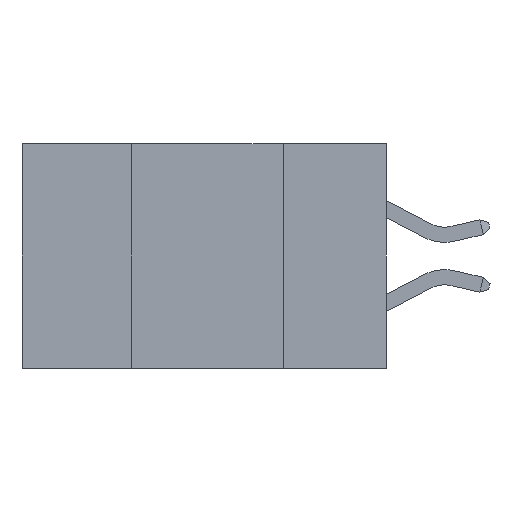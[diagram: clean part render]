
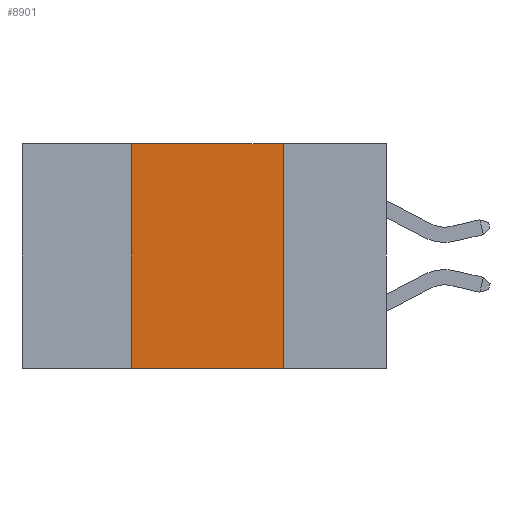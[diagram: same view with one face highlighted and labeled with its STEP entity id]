
A CAD part, left-side view. The second image highlights one B-rep face of the part: STEP entity #8901.
In plain terms, the highlighted planar face has unit normal (-1, 0, 0).
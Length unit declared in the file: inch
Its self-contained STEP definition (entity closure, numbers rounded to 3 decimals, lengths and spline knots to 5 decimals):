
#100 = DIRECTION ( 'NONE',  ( 0., -1., 0. ) ) ;
#317 = EDGE_LOOP ( 'NONE', ( #9134, #7067, #1886, #10419 ) ) ;
#601 = VERTEX_POINT ( 'NONE', #1994 ) ;
#633 = DIRECTION ( 'NONE',  ( 1., 0., 0. ) ) ;
#778 = VERTEX_POINT ( 'NONE', #4035 ) ;
#921 = VERTEX_POINT ( 'NONE', #9400 ) ;
#1886 = ORIENTED_EDGE ( 'NONE', *, *, #10093, .F. ) ;
#1994 = CARTESIAN_POINT ( 'NONE',  ( 0., 0.17, 0. ) ) ;
#2446 = CARTESIAN_POINT ( 'NONE',  ( 0., 0.42, -0.37 ) ) ;
#3532 = LINE ( 'NONE', #3844, #10837 ) ;
#3844 = CARTESIAN_POINT ( 'NONE',  ( 0., 0.6, -0.37 ) ) ;
#4035 = CARTESIAN_POINT ( 'NONE',  ( 0., 0.42, 0. ) ) ;
#5699 = CARTESIAN_POINT ( 'NONE',  ( 0., 0.6, 0. ) ) ;
#5722 = FACE_OUTER_BOUND ( 'NONE', #317, .T. ) ;
#5918 = EDGE_CURVE ( 'NONE', #6959, #921, #3532, .T. ) ;
#6034 = EDGE_CURVE ( 'NONE', #601, #921, #12149, .T. ) ;
#6339 = CARTESIAN_POINT ( 'NONE',  ( 0., 0.6, 0. ) ) ;
#6896 = EDGE_CURVE ( 'NONE', #778, #601, #9869, .T. ) ;
#6959 = VERTEX_POINT ( 'NONE', #2446 ) ;
#7067 = ORIENTED_EDGE ( 'NONE', *, *, #6896, .F. ) ;
#7763 = VECTOR ( 'NONE', #10952, 39.37008 ) ;
#8130 = DIRECTION ( 'NONE',  ( 0., 0., -1. ) ) ;
#8901 = ADVANCED_FACE ( 'NONE', ( #5722 ), #12241, .F. ) ;
#9134 = ORIENTED_EDGE ( 'NONE', *, *, #6034, .F. ) ;
#9400 = CARTESIAN_POINT ( 'NONE',  ( 0., 0.17, -0.37 ) ) ;
#9536 = VECTOR ( 'NONE', #12305, 39.37008 ) ;
#9706 = VECTOR ( 'NONE', #8130, 39.37008 ) ;
#9765 = AXIS2_PLACEMENT_3D ( 'NONE', #5699, #633, #10637 ) ;
#9869 = LINE ( 'NONE', #6339, #9536 ) ;
#10093 = EDGE_CURVE ( 'NONE', #6959, #778, #12498, .T. ) ;
#10419 = ORIENTED_EDGE ( 'NONE', *, *, #5918, .T. ) ;
#10637 = DIRECTION ( 'NONE',  ( 0., 0., -1. ) ) ;
#10837 = VECTOR ( 'NONE', #100, 39.37008 ) ;
#10952 = DIRECTION ( 'NONE',  ( 0., 0., 1. ) ) ;
#10991 = CARTESIAN_POINT ( 'NONE',  ( 0., 0.42, 0. ) ) ;
#12149 = LINE ( 'NONE', #12784, #9706 ) ;
#12241 = PLANE ( 'NONE',  #9765 ) ;
#12305 = DIRECTION ( 'NONE',  ( 0., -1., 0. ) ) ;
#12498 = LINE ( 'NONE', #10991, #7763 ) ;
#12784 = CARTESIAN_POINT ( 'NONE',  ( 0., 0.17, 0. ) ) ;
